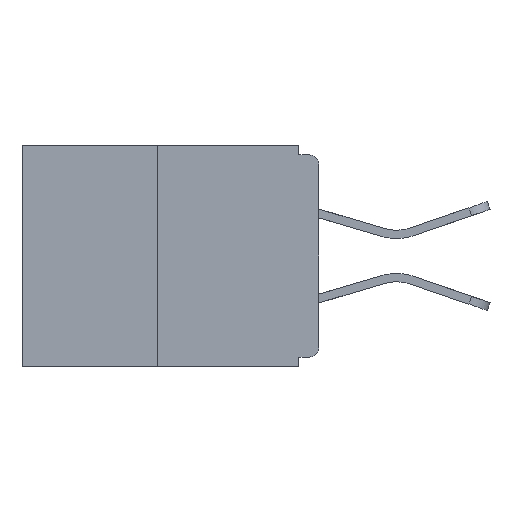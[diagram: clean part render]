
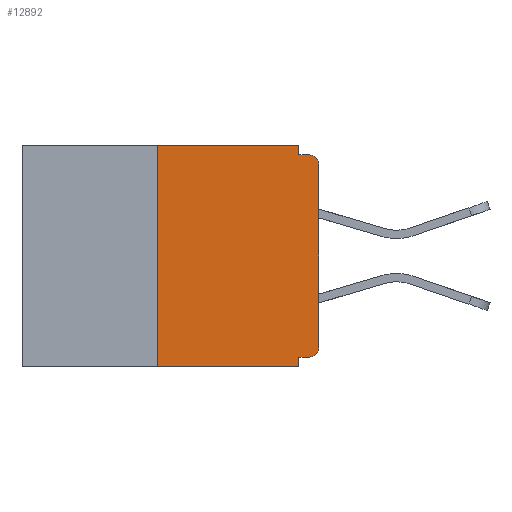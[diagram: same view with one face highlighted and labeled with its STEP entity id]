
A CAD part, left-side view. The second image highlights one B-rep face of the part: STEP entity #12892.
In plain terms, the highlighted planar face has unit normal (-1, 0, 0).
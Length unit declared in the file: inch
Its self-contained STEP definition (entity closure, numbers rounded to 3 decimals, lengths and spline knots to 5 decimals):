
#384 = VERTEX_POINT ( 'NONE', #4695 ) ;
#463 = ORIENTED_EDGE ( 'NONE', *, *, #9121, .F. ) ;
#528 = EDGE_CURVE ( 'NONE', #2840, #9097, #8423, .T. ) ;
#1082 = CARTESIAN_POINT ( 'NONE',  ( 0., 0.031, 0. ) ) ;
#1560 = CARTESIAN_POINT ( 'NONE',  ( 0., 0.031, -0.328 ) ) ;
#1563 = CARTESIAN_POINT ( 'NONE',  ( 0., 0., -0.328 ) ) ;
#1652 = LINE ( 'NONE', #1563, #8202 ) ;
#1897 = ORIENTED_EDGE ( 'NONE', *, *, #17995, .F. ) ;
#1898 = PLANE ( 'NONE',  #14424 ) ;
#1911 = CARTESIAN_POINT ( 'NONE',  ( 0., 0.25, 0. ) ) ;
#2017 = ORIENTED_EDGE ( 'NONE', *, *, #4783, .F. ) ;
#2119 = VECTOR ( 'NONE', #9966, 39.37008 ) ;
#2255 = CARTESIAN_POINT ( 'NONE',  ( 0., 0., -0.313 ) ) ;
#2440 = VECTOR ( 'NONE', #8526, 39.37008 ) ;
#2840 = VERTEX_POINT ( 'NONE', #12735 ) ;
#3257 = ORIENTED_EDGE ( 'NONE', *, *, #17757, .T. ) ;
#3293 = CARTESIAN_POINT ( 'NONE',  ( 0., 0.46, 0. ) ) ;
#3360 = EDGE_LOOP ( 'NONE', ( #9032, #1897, #11866, #8016, #11333, #9576, #3257, #8222, #463, #2017 ) ) ;
#3870 = CIRCLE ( 'NONE', #13109, 0.015 ) ;
#3901 = EDGE_CURVE ( 'NONE', #6089, #10650, #8221, .T. ) ;
#4119 = EDGE_CURVE ( 'NONE', #8932, #9382, #9104, .T. ) ;
#4217 = VECTOR ( 'NONE', #15861, 39.37008 ) ;
#4695 = CARTESIAN_POINT ( 'NONE',  ( 0., 0.015, -0.015 ) ) ;
#4783 = EDGE_CURVE ( 'NONE', #9097, #19623, #10115, .T. ) ;
#4902 = CARTESIAN_POINT ( 'NONE',  ( 0., 0., 0. ) ) ;
#5436 = CARTESIAN_POINT ( 'NONE',  ( 0., 0.015, -0.313 ) ) ;
#6037 = VERTEX_POINT ( 'NONE', #17588 ) ;
#6089 = VERTEX_POINT ( 'NONE', #11645 ) ;
#6559 = CARTESIAN_POINT ( 'NONE',  ( 0., 0.031, -0.343 ) ) ;
#7302 = LINE ( 'NONE', #14827, #2119 ) ;
#7383 = VERTEX_POINT ( 'NONE', #12448 ) ;
#7830 = DIRECTION ( 'NONE',  ( 0., 0., 1. ) ) ;
#8016 = ORIENTED_EDGE ( 'NONE', *, *, #4119, .F. ) ;
#8202 = VECTOR ( 'NONE', #15414, 39.37008 ) ;
#8221 = CIRCLE ( 'NONE', #15815, 0.015 ) ;
#8222 = ORIENTED_EDGE ( 'NONE', *, *, #12171, .T. ) ;
#8423 = LINE ( 'NONE', #9713, #4217 ) ;
#8526 = DIRECTION ( 'NONE',  ( 0., 0., -1. ) ) ;
#8932 = VERTEX_POINT ( 'NONE', #1560 ) ;
#9011 = LINE ( 'NONE', #10402, #15872 ) ;
#9032 = ORIENTED_EDGE ( 'NONE', *, *, #528, .F. ) ;
#9097 = VERTEX_POINT ( 'NONE', #1082 ) ;
#9104 = LINE ( 'NONE', #12160, #16441 ) ;
#9121 = EDGE_CURVE ( 'NONE', #19623, #384, #7302, .T. ) ;
#9382 = VERTEX_POINT ( 'NONE', #6559 ) ;
#9409 = DIRECTION ( 'NONE',  ( 1., 0., 0. ) ) ;
#9576 = ORIENTED_EDGE ( 'NONE', *, *, #3901, .T. ) ;
#9713 = CARTESIAN_POINT ( 'NONE',  ( 0., 0.46, 0. ) ) ;
#9966 = DIRECTION ( 'NONE',  ( 0., -1., 0. ) ) ;
#10115 = LINE ( 'NONE', #19307, #2440 ) ;
#10402 = CARTESIAN_POINT ( 'NONE',  ( 0., 0.46, -0.343 ) ) ;
#10650 = VERTEX_POINT ( 'NONE', #2255 ) ;
#11101 = EDGE_CURVE ( 'NONE', #6037, #9382, #9011, .T. ) ;
#11333 = ORIENTED_EDGE ( 'NONE', *, *, #16915, .F. ) ;
#11366 = VECTOR ( 'NONE', #7830, 39.37008 ) ;
#11624 = DIRECTION ( 'NONE',  ( 0., 0., -1. ) ) ;
#11645 = CARTESIAN_POINT ( 'NONE',  ( 0., 0.015, -0.328 ) ) ;
#11866 = ORIENTED_EDGE ( 'NONE', *, *, #11101, .T. ) ;
#12104 = LINE ( 'NONE', #4902, #11366 ) ;
#12160 = CARTESIAN_POINT ( 'NONE',  ( 0., 0.031, -0.343 ) ) ;
#12171 = EDGE_CURVE ( 'NONE', #7383, #384, #3870, .T. ) ;
#12448 = CARTESIAN_POINT ( 'NONE',  ( 0., 0., -0.03 ) ) ;
#12574 = CARTESIAN_POINT ( 'NONE',  ( 0., 0.015, -0.03 ) ) ;
#12735 = CARTESIAN_POINT ( 'NONE',  ( 0., 0.25, 0. ) ) ;
#12892 = ADVANCED_FACE ( 'NONE', ( #16735 ), #1898, .F. ) ;
#13012 = DIRECTION ( 'NONE',  ( -1., 0., 0. ) ) ;
#13109 = AXIS2_PLACEMENT_3D ( 'NONE', #12574, #16840, #17145 ) ;
#13470 = DIRECTION ( 'NONE',  ( 0., 0., -1. ) ) ;
#13593 = VECTOR ( 'NONE', #14690, 39.37008 ) ;
#14424 = AXIS2_PLACEMENT_3D ( 'NONE', #3293, #9409, #18506 ) ;
#14690 = DIRECTION ( 'NONE',  ( 0., 0., 1. ) ) ;
#14827 = CARTESIAN_POINT ( 'NONE',  ( 0., 0., -0.015 ) ) ;
#15414 = DIRECTION ( 'NONE',  ( 0., 1., 0. ) ) ;
#15574 = LINE ( 'NONE', #1911, #13593 ) ;
#15815 = AXIS2_PLACEMENT_3D ( 'NONE', #5436, #13012, #11624 ) ;
#15861 = DIRECTION ( 'NONE',  ( 0., -1., 0. ) ) ;
#15872 = VECTOR ( 'NONE', #18014, 39.37008 ) ;
#16441 = VECTOR ( 'NONE', #13470, 39.37008 ) ;
#16735 = FACE_OUTER_BOUND ( 'NONE', #3360, .T. ) ;
#16840 = DIRECTION ( 'NONE',  ( -1., 0., 0. ) ) ;
#16915 = EDGE_CURVE ( 'NONE', #6089, #8932, #1652, .T. ) ;
#17145 = DIRECTION ( 'NONE',  ( 0., 0., -1. ) ) ;
#17588 = CARTESIAN_POINT ( 'NONE',  ( 0., 0.25, -0.343 ) ) ;
#17757 = EDGE_CURVE ( 'NONE', #10650, #7383, #12104, .T. ) ;
#17995 = EDGE_CURVE ( 'NONE', #6037, #2840, #15574, .T. ) ;
#18014 = DIRECTION ( 'NONE',  ( 0., -1., 0. ) ) ;
#18506 = DIRECTION ( 'NONE',  ( 0., 0., -1. ) ) ;
#19307 = CARTESIAN_POINT ( 'NONE',  ( 0., 0.031, 0. ) ) ;
#19429 = CARTESIAN_POINT ( 'NONE',  ( 0., 0.031, -0.015 ) ) ;
#19623 = VERTEX_POINT ( 'NONE', #19429 ) ;
